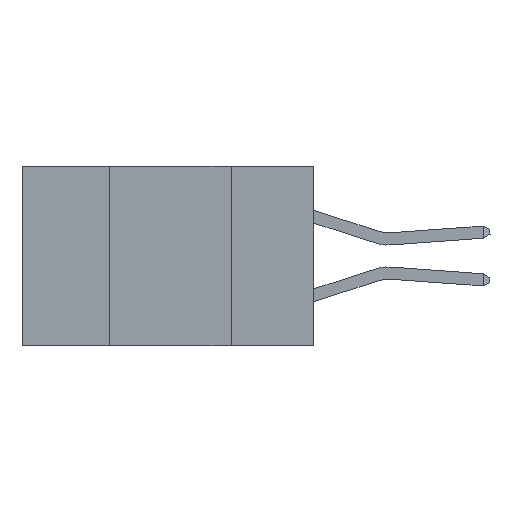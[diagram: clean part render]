
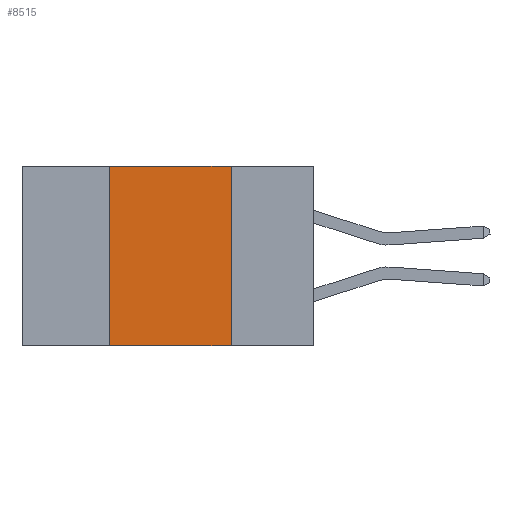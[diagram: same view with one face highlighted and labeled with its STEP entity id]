
A CAD part, left-side view. The second image highlights one B-rep face of the part: STEP entity #8515.
In plain terms, the highlighted planar face has unit normal (-1, 0, 0).
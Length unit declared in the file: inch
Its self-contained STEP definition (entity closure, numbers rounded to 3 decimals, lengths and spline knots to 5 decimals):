
#14 = EDGE_CURVE ( 'NONE', #2489, #4679, #9142, .T. ) ;
#389 = DIRECTION ( 'NONE',  ( 0., 0., -1. ) ) ;
#830 = VERTEX_POINT ( 'NONE', #11902 ) ;
#1211 = EDGE_CURVE ( 'NONE', #12752, #4679, #5135, .T. ) ;
#2489 = VERTEX_POINT ( 'NONE', #5268 ) ;
#2830 = EDGE_CURVE ( 'NONE', #830, #2489, #7357, .T. ) ;
#3208 = DIRECTION ( 'NONE',  ( 0., -1., 0. ) ) ;
#3969 = EDGE_LOOP ( 'NONE', ( #11932, #7939, #14823, #14057 ) ) ;
#4443 = CARTESIAN_POINT ( 'NONE',  ( 0., 0.6, -0.37 ) ) ;
#4679 = VERTEX_POINT ( 'NONE', #8363 ) ;
#4986 = CARTESIAN_POINT ( 'NONE',  ( 0., 0.17, 0. ) ) ;
#5135 = LINE ( 'NONE', #4443, #14152 ) ;
#5268 = CARTESIAN_POINT ( 'NONE',  ( 0., 0.17, 0. ) ) ;
#5304 = EDGE_CURVE ( 'NONE', #12752, #830, #10888, .T. ) ;
#5738 = AXIS2_PLACEMENT_3D ( 'NONE', #14270, #7371, #389 ) ;
#6173 = PLANE ( 'NONE',  #5738 ) ;
#6214 = DIRECTION ( 'NONE',  ( 0., 0., -1. ) ) ;
#6639 = DIRECTION ( 'NONE',  ( 0., 0., 1. ) ) ;
#7357 = LINE ( 'NONE', #7416, #14736 ) ;
#7371 = DIRECTION ( 'NONE',  ( 1., 0., 0. ) ) ;
#7416 = CARTESIAN_POINT ( 'NONE',  ( 0., 0.6, 0. ) ) ;
#7939 = ORIENTED_EDGE ( 'NONE', *, *, #2830, .F. ) ;
#7955 = CARTESIAN_POINT ( 'NONE',  ( 0., 0.42, -0.37 ) ) ;
#8363 = CARTESIAN_POINT ( 'NONE',  ( 0., 0.17, -0.37 ) ) ;
#8515 = ADVANCED_FACE ( 'NONE', ( #8745 ), #6173, .F. ) ;
#8745 = FACE_OUTER_BOUND ( 'NONE', #3969, .T. ) ;
#9142 = LINE ( 'NONE', #4986, #12185 ) ;
#10888 = LINE ( 'NONE', #11146, #13942 ) ;
#11146 = CARTESIAN_POINT ( 'NONE',  ( 0., 0.42, 0. ) ) ;
#11902 = CARTESIAN_POINT ( 'NONE',  ( 0., 0.42, 0. ) ) ;
#11932 = ORIENTED_EDGE ( 'NONE', *, *, #14, .F. ) ;
#12185 = VECTOR ( 'NONE', #6214, 39.37008 ) ;
#12752 = VERTEX_POINT ( 'NONE', #7955 ) ;
#13475 = DIRECTION ( 'NONE',  ( 0., -1., 0. ) ) ;
#13942 = VECTOR ( 'NONE', #6639, 39.37008 ) ;
#14057 = ORIENTED_EDGE ( 'NONE', *, *, #1211, .T. ) ;
#14152 = VECTOR ( 'NONE', #3208, 39.37008 ) ;
#14270 = CARTESIAN_POINT ( 'NONE',  ( 0., 0.6, 0. ) ) ;
#14736 = VECTOR ( 'NONE', #13475, 39.37008 ) ;
#14823 = ORIENTED_EDGE ( 'NONE', *, *, #5304, .F. ) ;
